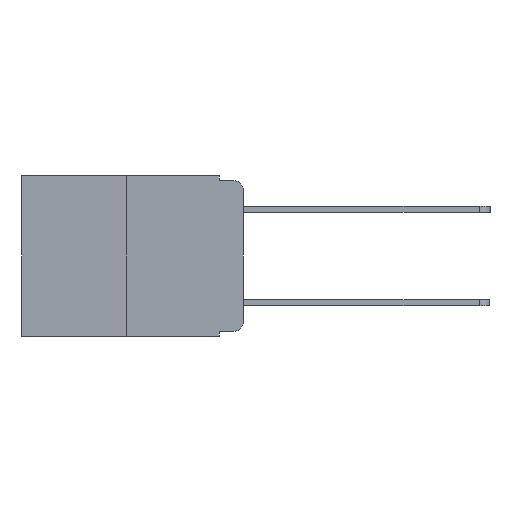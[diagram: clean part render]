
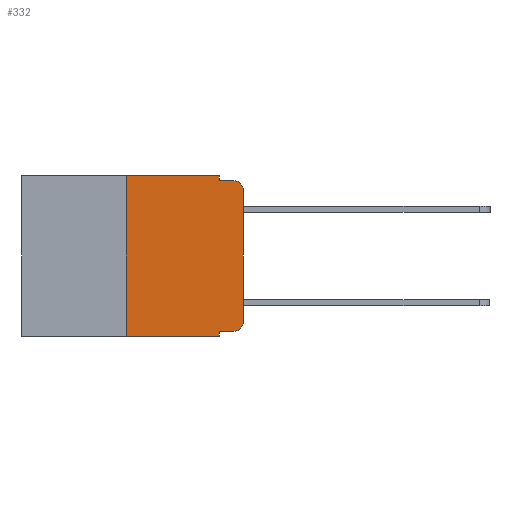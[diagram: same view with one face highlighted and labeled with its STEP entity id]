
A CAD part, left-side view. The second image highlights one B-rep face of the part: STEP entity #332.
In plain terms, the highlighted planar face has unit normal (-1, 0, 0).
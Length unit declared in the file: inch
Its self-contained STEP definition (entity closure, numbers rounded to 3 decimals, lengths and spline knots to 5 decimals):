
#332 = ADVANCED_FACE ( 'NONE', ( #4199 ), #16517, .F. ) ;
#643 = DIRECTION ( 'NONE',  ( 0., -1., 0. ) ) ;
#855 = CIRCLE ( 'NONE', #13007, 0.02 ) ;
#965 = DIRECTION ( 'NONE',  ( 0., 0., -1. ) ) ;
#985 = VECTOR ( 'NONE', #10517, 39.37008 ) ;
#1763 = CARTESIAN_POINT ( 'NONE',  ( 0., 0.051, -0.01 ) ) ;
#2082 = ORIENTED_EDGE ( 'NONE', *, *, #14793, .T. ) ;
#2211 = CARTESIAN_POINT ( 'NONE',  ( 0., 0.051, 0. ) ) ;
#2442 = EDGE_CURVE ( 'NONE', #12305, #7065, #15419, .T. ) ;
#2505 = CARTESIAN_POINT ( 'NONE',  ( 0., 0.051, 0. ) ) ;
#3286 = VERTEX_POINT ( 'NONE', #2211 ) ;
#3307 = CARTESIAN_POINT ( 'NONE',  ( 0., 0.25, 0. ) ) ;
#3352 = VERTEX_POINT ( 'NONE', #8223 ) ;
#3652 = CARTESIAN_POINT ( 'NONE',  ( 0., 0.051, -0.333 ) ) ;
#3749 = VERTEX_POINT ( 'NONE', #1763 ) ;
#3906 = VECTOR ( 'NONE', #4731, 39.37008 ) ;
#4199 = FACE_OUTER_BOUND ( 'NONE', #5669, .T. ) ;
#4229 = ORIENTED_EDGE ( 'NONE', *, *, #16183, .F. ) ;
#4386 = CARTESIAN_POINT ( 'NONE',  ( 0., 0.02, -0.03 ) ) ;
#4694 = CARTESIAN_POINT ( 'NONE',  ( 0., 0.051, -0.333 ) ) ;
#4731 = DIRECTION ( 'NONE',  ( 0., 0., 1. ) ) ;
#4914 = CARTESIAN_POINT ( 'NONE',  ( 0., 0.051, -0.01 ) ) ;
#5056 = DIRECTION ( 'NONE',  ( 0., -1., 0. ) ) ;
#5289 = VERTEX_POINT ( 'NONE', #15347 ) ;
#5320 = VERTEX_POINT ( 'NONE', #9568 ) ;
#5464 = VECTOR ( 'NONE', #16150, 39.37008 ) ;
#5669 = EDGE_LOOP ( 'NONE', ( #13341, #8866, #15758, #8490, #4229, #6276, #2082, #6679, #9684, #13372 ) ) ;
#5701 = DIRECTION ( 'NONE',  ( 0., 0., -1. ) ) ;
#6276 = ORIENTED_EDGE ( 'NONE', *, *, #11128, .F. ) ;
#6385 = CARTESIAN_POINT ( 'NONE',  ( 0., 0.473, -0.343 ) ) ;
#6423 = EDGE_CURVE ( 'NONE', #12305, #11487, #11733, .T. ) ;
#6640 = VERTEX_POINT ( 'NONE', #16554 ) ;
#6679 = ORIENTED_EDGE ( 'NONE', *, *, #2442, .F. ) ;
#7051 = VERTEX_POINT ( 'NONE', #15981 ) ;
#7065 = VERTEX_POINT ( 'NONE', #14840 ) ;
#7882 = CARTESIAN_POINT ( 'NONE',  ( 0., 0.02, -0.333 ) ) ;
#8040 = DIRECTION ( 'NONE',  ( 0., -1., 0. ) ) ;
#8155 = EDGE_CURVE ( 'NONE', #11487, #7051, #855, .T. ) ;
#8223 = CARTESIAN_POINT ( 'NONE',  ( 0., 0.25, -0.343 ) ) ;
#8375 = CARTESIAN_POINT ( 'NONE',  ( 0., 0.473, 0. ) ) ;
#8490 = ORIENTED_EDGE ( 'NONE', *, *, #11881, .F. ) ;
#8866 = ORIENTED_EDGE ( 'NONE', *, *, #12946, .T. ) ;
#8931 = LINE ( 'NONE', #6385, #15100 ) ;
#9019 = VECTOR ( 'NONE', #8040, 39.37008 ) ;
#9185 = LINE ( 'NONE', #2505, #985 ) ;
#9225 = DIRECTION ( 'NONE',  ( -1., 0., 0. ) ) ;
#9316 = CARTESIAN_POINT ( 'NONE',  ( 0., 0.473, 0. ) ) ;
#9568 = CARTESIAN_POINT ( 'NONE',  ( 0., 0.02, -0.01 ) ) ;
#9684 = ORIENTED_EDGE ( 'NONE', *, *, #6423, .T. ) ;
#9821 = VECTOR ( 'NONE', #16461, 39.37008 ) ;
#9874 = DIRECTION ( 'NONE',  ( 1., 0., 0. ) ) ;
#10517 = DIRECTION ( 'NONE',  ( 0., 0., -1. ) ) ;
#10537 = EDGE_CURVE ( 'NONE', #3749, #5320, #16090, .T. ) ;
#11031 = LINE ( 'NONE', #12925, #9821 ) ;
#11128 = EDGE_CURVE ( 'NONE', #3352, #5289, #11214, .T. ) ;
#11214 = LINE ( 'NONE', #3307, #3906 ) ;
#11353 = VECTOR ( 'NONE', #5056, 39.37008 ) ;
#11487 = VERTEX_POINT ( 'NONE', #7882 ) ;
#11685 = DIRECTION ( 'NONE',  ( 0., 0., -1. ) ) ;
#11733 = LINE ( 'NONE', #3652, #11353 ) ;
#11881 = EDGE_CURVE ( 'NONE', #3286, #3749, #9185, .T. ) ;
#12305 = VERTEX_POINT ( 'NONE', #4694 ) ;
#12925 = CARTESIAN_POINT ( 'NONE',  ( 0., 0., 0. ) ) ;
#12931 = VECTOR ( 'NONE', #13745, 39.37008 ) ;
#12946 = EDGE_CURVE ( 'NONE', #6640, #5320, #13619, .T. ) ;
#13007 = AXIS2_PLACEMENT_3D ( 'NONE', #16520, #9225, #965 ) ;
#13102 = LINE ( 'NONE', #9316, #9019 ) ;
#13266 = DIRECTION ( 'NONE',  ( -1., 0., 0. ) ) ;
#13341 = ORIENTED_EDGE ( 'NONE', *, *, #16124, .T. ) ;
#13372 = ORIENTED_EDGE ( 'NONE', *, *, #8155, .T. ) ;
#13541 = CARTESIAN_POINT ( 'NONE',  ( 0., 0.051, 0. ) ) ;
#13619 = CIRCLE ( 'NONE', #16333, 0.02 ) ;
#13745 = DIRECTION ( 'NONE',  ( 0., -1., 0. ) ) ;
#14793 = EDGE_CURVE ( 'NONE', #3352, #7065, #8931, .T. ) ;
#14840 = CARTESIAN_POINT ( 'NONE',  ( 0., 0.051, -0.343 ) ) ;
#15100 = VECTOR ( 'NONE', #643, 39.37008 ) ;
#15347 = CARTESIAN_POINT ( 'NONE',  ( 0., 0.25, 0. ) ) ;
#15419 = LINE ( 'NONE', #13541, #5464 ) ;
#15758 = ORIENTED_EDGE ( 'NONE', *, *, #10537, .F. ) ;
#15981 = CARTESIAN_POINT ( 'NONE',  ( 0., 0., -0.313 ) ) ;
#16090 = LINE ( 'NONE', #4914, #12931 ) ;
#16124 = EDGE_CURVE ( 'NONE', #7051, #6640, #11031, .T. ) ;
#16150 = DIRECTION ( 'NONE',  ( 0., 0., -1. ) ) ;
#16183 = EDGE_CURVE ( 'NONE', #5289, #3286, #13102, .T. ) ;
#16187 = AXIS2_PLACEMENT_3D ( 'NONE', #8375, #9874, #11685 ) ;
#16333 = AXIS2_PLACEMENT_3D ( 'NONE', #4386, #13266, #5701 ) ;
#16461 = DIRECTION ( 'NONE',  ( 0., 0., 1. ) ) ;
#16517 = PLANE ( 'NONE',  #16187 ) ;
#16520 = CARTESIAN_POINT ( 'NONE',  ( 0., 0.02, -0.313 ) ) ;
#16554 = CARTESIAN_POINT ( 'NONE',  ( 0., 0., -0.03 ) ) ;
